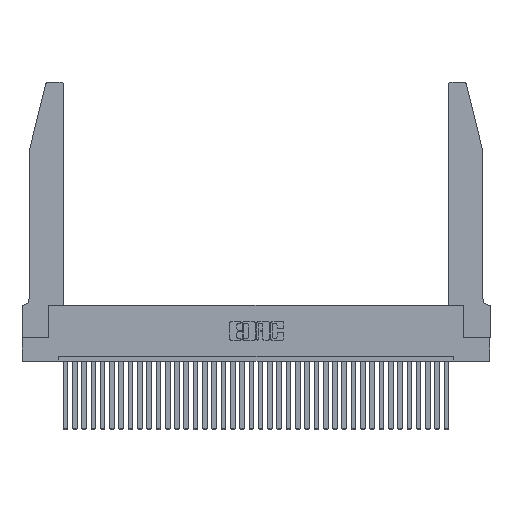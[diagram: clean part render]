
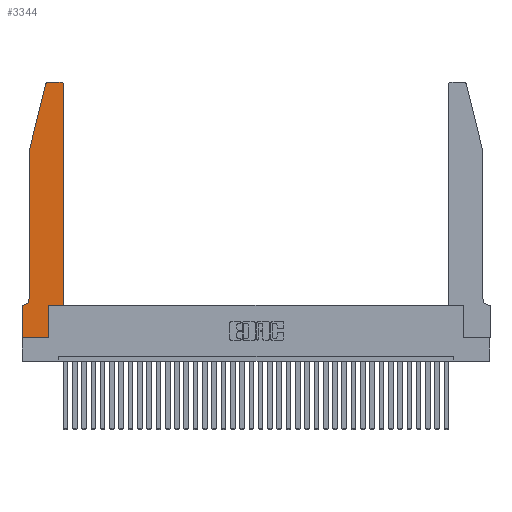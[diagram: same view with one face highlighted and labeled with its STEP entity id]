
A CAD part, top view. The second image highlights one B-rep face of the part: STEP entity #3344.
In plain terms, the highlighted planar face has unit normal (0, 0, 1).
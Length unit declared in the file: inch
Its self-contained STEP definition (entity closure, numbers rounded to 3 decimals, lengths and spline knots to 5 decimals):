
#238 = DIRECTION ( 'NONE',  ( -1., 0., 0. ) ) ;
#294 = VECTOR ( 'NONE', #18408, 39.37008 ) ;
#427 = EDGE_CURVE ( 'NONE', #1986, #19759, #9049, .T. ) ;
#555 = EDGE_LOOP ( 'NONE', ( #6357, #20096, #32388, #30071, #13917, #7071, #33436, #28751, #1743, #9791, #35018, #11824 ) ) ;
#1743 = ORIENTED_EDGE ( 'NONE', *, *, #427, .T. ) ;
#1812 = CARTESIAN_POINT ( 'NONE',  ( 0., 0., 0.37 ) ) ;
#1986 = VERTEX_POINT ( 'NONE', #6579 ) ;
#2511 = CARTESIAN_POINT ( 'NONE',  ( 0.4205, 2.72, 0.37 ) ) ;
#3152 = LINE ( 'NONE', #10175, #24087 ) ;
#3344 = ADVANCED_FACE ( 'NONE', ( #25851 ), #7349, .T. ) ;
#3366 = DIRECTION ( 'NONE',  ( 0., -1., 0. ) ) ;
#4870 = CARTESIAN_POINT ( 'NONE',  ( 0.2865, 0.35, 0.37 ) ) ;
#5585 = LINE ( 'NONE', #15507, #30096 ) ;
#5622 = CIRCLE ( 'NONE', #21588, 0.07 ) ;
#5628 = EDGE_CURVE ( 'NONE', #31632, #34269, #5622, .T. ) ;
#5646 = CARTESIAN_POINT ( 'NONE',  ( 0.4505, 0.35, 0.37 ) ) ;
#6001 = CARTESIAN_POINT ( 'NONE',  ( 0.284, 2.72, 0.37 ) ) ;
#6357 = ORIENTED_EDGE ( 'NONE', *, *, #32897, .T. ) ;
#6579 = CARTESIAN_POINT ( 'NONE',  ( 0.2865, 0., 0.37 ) ) ;
#7049 = DIRECTION ( 'NONE',  ( 1., 0., 0. ) ) ;
#7071 = ORIENTED_EDGE ( 'NONE', *, *, #9195, .T. ) ;
#7133 = CARTESIAN_POINT ( 'NONE',  ( 0.0755, 0.35, 0.37 ) ) ;
#7349 = PLANE ( 'NONE',  #23782 ) ;
#7889 = VERTEX_POINT ( 'NONE', #28220 ) ;
#8035 = CARTESIAN_POINT ( 'NONE',  ( 0.0755, 2., 0.37 ) ) ;
#8445 = DIRECTION ( 'NONE',  ( 1., 0., 0. ) ) ;
#9049 = LINE ( 'NONE', #4870, #294 ) ;
#9195 = EDGE_CURVE ( 'NONE', #34269, #20743, #12427, .T. ) ;
#9550 = EDGE_CURVE ( 'NONE', #19759, #16495, #17115, .T. ) ;
#9791 = ORIENTED_EDGE ( 'NONE', *, *, #9550, .T. ) ;
#10058 = DIRECTION ( 'NONE',  ( 0., 0., 1. ) ) ;
#10175 = CARTESIAN_POINT ( 'NONE',  ( 0.0755, 2., 0.37 ) ) ;
#11606 = DIRECTION ( 'NONE',  ( -0.239, -0.971, 0. ) ) ;
#11667 = DIRECTION ( 'NONE',  ( 1., 0., 0. ) ) ;
#11824 = ORIENTED_EDGE ( 'NONE', *, *, #33569, .T. ) ;
#12396 = VECTOR ( 'NONE', #8445, 39.37008 ) ;
#12427 = LINE ( 'NONE', #7133, #29393 ) ;
#12970 = VERTEX_POINT ( 'NONE', #18718 ) ;
#13262 = DIRECTION ( 'NONE',  ( 1., 0., 0. ) ) ;
#13518 = VERTEX_POINT ( 'NONE', #27115 ) ;
#13917 = ORIENTED_EDGE ( 'NONE', *, *, #5628, .T. ) ;
#13918 = VERTEX_POINT ( 'NONE', #33633 ) ;
#14038 = VECTOR ( 'NONE', #3366, 39.37008 ) ;
#14217 = DIRECTION ( 'NONE',  ( 0., 0., -1. ) ) ;
#15507 = CARTESIAN_POINT ( 'NONE',  ( 0.2605, 2.75, 0.37 ) ) ;
#15658 = CARTESIAN_POINT ( 'NONE',  ( 0.284, 2.75, 0.37 ) ) ;
#15832 = EDGE_CURVE ( 'NONE', #7889, #31632, #3152, .T. ) ;
#15932 = CARTESIAN_POINT ( 'NONE',  ( 0.4505, 0.35, 0.37 ) ) ;
#16495 = VERTEX_POINT ( 'NONE', #30413 ) ;
#17115 = LINE ( 'NONE', #5646, #12396 ) ;
#17348 = EDGE_CURVE ( 'NONE', #20743, #35639, #28863, .T. ) ;
#18127 = EDGE_CURVE ( 'NONE', #18389, #12970, #35789, .T. ) ;
#18389 = VERTEX_POINT ( 'NONE', #15658 ) ;
#18408 = DIRECTION ( 'NONE',  ( 0., 1., 0. ) ) ;
#18718 = CARTESIAN_POINT ( 'NONE',  ( 0.25487, 2.72718, 0.37 ) ) ;
#19354 = DIRECTION ( 'NONE',  ( 1., 0., 0. ) ) ;
#19759 = VERTEX_POINT ( 'NONE', #29465 ) ;
#20078 = CARTESIAN_POINT ( 'NONE',  ( 0., 0., 0.37 ) ) ;
#20096 = ORIENTED_EDGE ( 'NONE', *, *, #18127, .T. ) ;
#20299 = LINE ( 'NONE', #15932, #35991 ) ;
#20696 = VECTOR ( 'NONE', #11606, 39.37008 ) ;
#20743 = VERTEX_POINT ( 'NONE', #29516 ) ;
#21180 = DIRECTION ( 'NONE',  ( 0., 1., 0. ) ) ;
#21288 = DIRECTION ( 'NONE',  ( -1., 0., 0. ) ) ;
#21550 = EDGE_CURVE ( 'NONE', #12970, #7889, #35530, .T. ) ;
#21588 = AXIS2_PLACEMENT_3D ( 'NONE', #33731, #14217, #238 ) ;
#22342 = CARTESIAN_POINT ( 'NONE',  ( 0.0055, 0.35, 0.37 ) ) ;
#23353 = AXIS2_PLACEMENT_3D ( 'NONE', #2511, #33146, #19354 ) ;
#23782 = AXIS2_PLACEMENT_3D ( 'NONE', #26775, #10058, #13262 ) ;
#23885 = DIRECTION ( 'NONE',  ( -1., 0., 0. ) ) ;
#24087 = VECTOR ( 'NONE', #26634, 39.37008 ) ;
#24807 = CARTESIAN_POINT ( 'NONE',  ( 0., 0., 0.37 ) ) ;
#24944 = EDGE_CURVE ( 'NONE', #16495, #13518, #20299, .T. ) ;
#25516 = DIRECTION ( 'NONE',  ( 0., 0., 1. ) ) ;
#25845 = LINE ( 'NONE', #1812, #27210 ) ;
#25851 = FACE_OUTER_BOUND ( 'NONE', #555, .T. ) ;
#26113 = EDGE_CURVE ( 'NONE', #35639, #1986, #25845, .T. ) ;
#26497 = AXIS2_PLACEMENT_3D ( 'NONE', #6001, #25516, #11667 ) ;
#26634 = DIRECTION ( 'NONE',  ( 0., -1., 0. ) ) ;
#26775 = CARTESIAN_POINT ( 'NONE',  ( 0., 0.35, 0.37 ) ) ;
#27115 = CARTESIAN_POINT ( 'NONE',  ( 0.4505, 2.72, 0.37 ) ) ;
#27210 = VECTOR ( 'NONE', #7049, 39.37008 ) ;
#28220 = CARTESIAN_POINT ( 'NONE',  ( 0.0755, 2., 0.37 ) ) ;
#28751 = ORIENTED_EDGE ( 'NONE', *, *, #26113, .T. ) ;
#28863 = LINE ( 'NONE', #20078, #14038 ) ;
#29133 = CIRCLE ( 'NONE', #23353, 0.03 ) ;
#29393 = VECTOR ( 'NONE', #21288, 39.37008 ) ;
#29465 = CARTESIAN_POINT ( 'NONE',  ( 0.2865, 0.35, 0.37 ) ) ;
#29516 = CARTESIAN_POINT ( 'NONE',  ( 0., 0.35, 0.37 ) ) ;
#30071 = ORIENTED_EDGE ( 'NONE', *, *, #15832, .T. ) ;
#30096 = VECTOR ( 'NONE', #23885, 39.37008 ) ;
#30413 = CARTESIAN_POINT ( 'NONE',  ( 0.4505, 0.35, 0.37 ) ) ;
#31632 = VERTEX_POINT ( 'NONE', #33344 ) ;
#32388 = ORIENTED_EDGE ( 'NONE', *, *, #21550, .T. ) ;
#32897 = EDGE_CURVE ( 'NONE', #13918, #18389, #5585, .T. ) ;
#33146 = DIRECTION ( 'NONE',  ( 0., 0., 1. ) ) ;
#33344 = CARTESIAN_POINT ( 'NONE',  ( 0.0755, 0.42, 0.37 ) ) ;
#33436 = ORIENTED_EDGE ( 'NONE', *, *, #17348, .T. ) ;
#33569 = EDGE_CURVE ( 'NONE', #13518, #13918, #29133, .T. ) ;
#33633 = CARTESIAN_POINT ( 'NONE',  ( 0.4205, 2.75, 0.37 ) ) ;
#33731 = CARTESIAN_POINT ( 'NONE',  ( 0.0055, 0.42, 0.37 ) ) ;
#34269 = VERTEX_POINT ( 'NONE', #22342 ) ;
#35018 = ORIENTED_EDGE ( 'NONE', *, *, #24944, .T. ) ;
#35530 = LINE ( 'NONE', #8035, #20696 ) ;
#35639 = VERTEX_POINT ( 'NONE', #24807 ) ;
#35789 = CIRCLE ( 'NONE', #26497, 0.03 ) ;
#35991 = VECTOR ( 'NONE', #21180, 39.37008 ) ;
